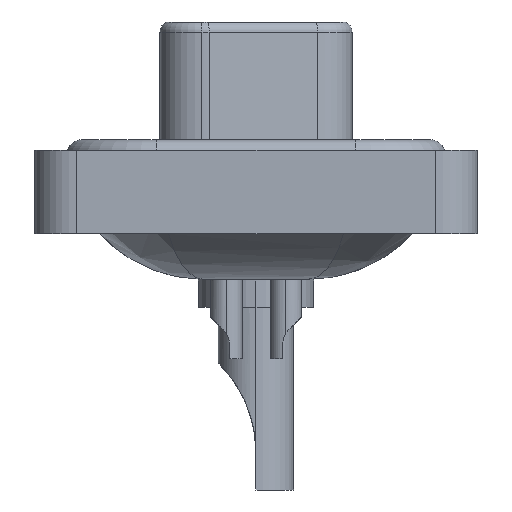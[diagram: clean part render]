
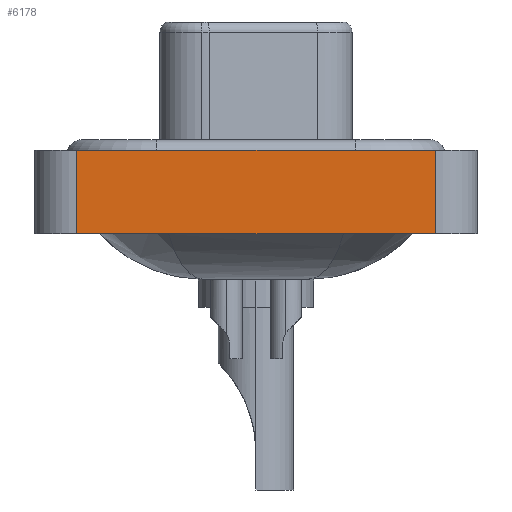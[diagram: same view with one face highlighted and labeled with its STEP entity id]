
A CAD part, left-side view. The second image highlights one B-rep face of the part: STEP entity #6178.
In plain terms, the highlighted planar face has unit normal (-1, 0, 0).
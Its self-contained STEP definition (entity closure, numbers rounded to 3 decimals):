
#281 = CARTESIAN_POINT ( 'NONE',  ( -7.25, -8.55, 0.4 ) ) ;
#367 = DIRECTION ( 'NONE',  ( 0., 0., 1. ) ) ;
#1245 = EDGE_CURVE ( 'NONE', #12797, #10068, #17889, .T. ) ;
#1804 = DIRECTION ( 'NONE',  ( 0., -1., 0. ) ) ;
#2492 = VECTOR ( 'NONE', #367, 1000. ) ;
#2771 = EDGE_LOOP ( 'NONE', ( #3474, #10672, #6886, #9989 ) ) ;
#3474 = ORIENTED_EDGE ( 'NONE', *, *, #7026, .T. ) ;
#3906 = CARTESIAN_POINT ( 'NONE',  ( -7.25, -8.55, 0.4 ) ) ;
#3999 = LINE ( 'NONE', #3906, #11237 ) ;
#4305 = VERTEX_POINT ( 'NONE', #281 ) ;
#4346 = AXIS2_PLACEMENT_3D ( 'NONE', #9950, #11511, #12957 ) ;
#4731 = LINE ( 'NONE', #10257, #2492 ) ;
#5166 = VECTOR ( 'NONE', #1804, 1000. ) ;
#6178 = ADVANCED_FACE ( 'NONE', ( #7407 ), #15415, .T. ) ;
#6886 = ORIENTED_EDGE ( 'NONE', *, *, #13020, .F. ) ;
#7026 = EDGE_CURVE ( 'NONE', #10068, #4305, #17893, .T. ) ;
#7174 = CARTESIAN_POINT ( 'NONE',  ( -7.25, -8.55, -3.6 ) ) ;
#7407 = FACE_OUTER_BOUND ( 'NONE', #2771, .T. ) ;
#9950 = CARTESIAN_POINT ( 'NONE',  ( -7.25, -8.55, -3.6 ) ) ;
#9989 = ORIENTED_EDGE ( 'NONE', *, *, #1245, .T. ) ;
#10068 = VERTEX_POINT ( 'NONE', #7174 ) ;
#10257 = CARTESIAN_POINT ( 'NONE',  ( -7.25, 8.55, -3.6 ) ) ;
#10375 = EDGE_CURVE ( 'NONE', #13127, #4305, #3999, .T. ) ;
#10672 = ORIENTED_EDGE ( 'NONE', *, *, #10375, .F. ) ;
#11237 = VECTOR ( 'NONE', #12351, 1000. ) ;
#11511 = DIRECTION ( 'NONE',  ( -1., 0., 0. ) ) ;
#11731 = CARTESIAN_POINT ( 'NONE',  ( -7.25, 8.55, 0.4 ) ) ;
#12296 = CARTESIAN_POINT ( 'NONE',  ( -7.25, 8.55, -3.6 ) ) ;
#12351 = DIRECTION ( 'NONE',  ( 0., -1., 0. ) ) ;
#12797 = VERTEX_POINT ( 'NONE', #12296 ) ;
#12957 = DIRECTION ( 'NONE',  ( 0., 0., 1. ) ) ;
#13020 = EDGE_CURVE ( 'NONE', #12797, #13127, #4731, .T. ) ;
#13127 = VERTEX_POINT ( 'NONE', #11731 ) ;
#14931 = CARTESIAN_POINT ( 'NONE',  ( -7.25, -8.55, -3.6 ) ) ;
#15415 = PLANE ( 'NONE',  #4346 ) ;
#16361 = DIRECTION ( 'NONE',  ( 0., 0., 1. ) ) ;
#16534 = CARTESIAN_POINT ( 'NONE',  ( -7.25, -8.55, -3.6 ) ) ;
#17372 = VECTOR ( 'NONE', #16361, 1000. ) ;
#17889 = LINE ( 'NONE', #16534, #5166 ) ;
#17893 = LINE ( 'NONE', #14931, #17372 ) ;
